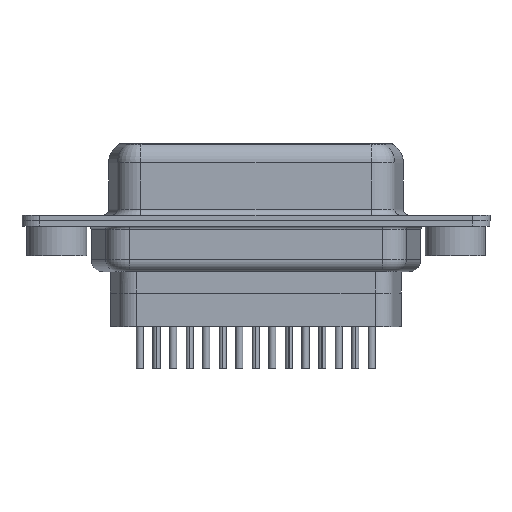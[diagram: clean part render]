
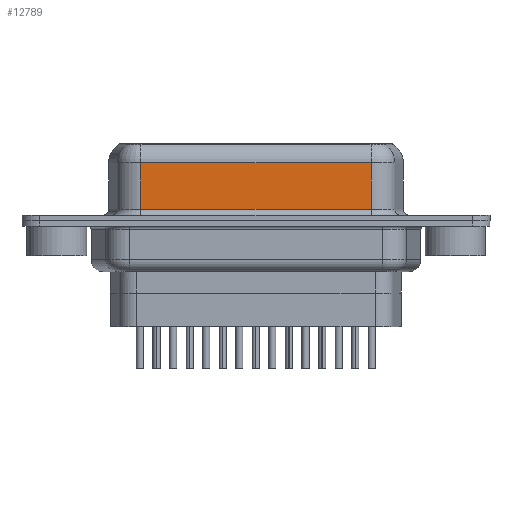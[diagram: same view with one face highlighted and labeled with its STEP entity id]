
A CAD part, front view. The second image highlights one B-rep face of the part: STEP entity #12789.
In plain terms, the highlighted planar face has unit normal (0, -1, 0).
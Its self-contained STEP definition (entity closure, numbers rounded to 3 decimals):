
#417 = ORIENTED_EDGE ( 'NONE', *, *, #6858, .T. ) ;
#1581 = VERTEX_POINT ( 'NONE', #16875 ) ;
#2414 = VERTEX_POINT ( 'NONE', #3272 ) ;
#3272 = CARTESIAN_POINT ( 'NONE',  ( 7.023, -3.95, 0.95 ) ) ;
#3431 = DIRECTION ( 'NONE',  ( -1., 0., 0. ) ) ;
#3705 = CARTESIAN_POINT ( 'NONE',  ( 26.297, -3.95, 4.85 ) ) ;
#6474 = CARTESIAN_POINT ( 'NONE',  ( 26.297, -3.95, 6.6 ) ) ;
#6818 = DIRECTION ( 'NONE',  ( 1., 0., 0. ) ) ;
#6858 = EDGE_CURVE ( 'NONE', #17644, #1581, #11317, .T. ) ;
#7338 = EDGE_CURVE ( 'NONE', #2414, #22537, #8996, .T. ) ;
#7809 = CARTESIAN_POINT ( 'NONE',  ( 7.023, -3.95, 6.6 ) ) ;
#8597 = DIRECTION ( 'NONE',  ( 0., 1., 0. ) ) ;
#8996 = LINE ( 'NONE', #24729, #21390 ) ;
#9971 = EDGE_CURVE ( 'NONE', #1581, #2414, #13467, .T. ) ;
#10147 = ORIENTED_EDGE ( 'NONE', *, *, #7338, .T. ) ;
#10273 = VECTOR ( 'NONE', #3431, 1000. ) ;
#10531 = FACE_OUTER_BOUND ( 'NONE', #23158, .T. ) ;
#11317 = LINE ( 'NONE', #3705, #10273 ) ;
#11361 = CARTESIAN_POINT ( 'NONE',  ( 26.297, -3.95, 4.85 ) ) ;
#11907 = CARTESIAN_POINT ( 'NONE',  ( 26.297, -3.95, 0.95 ) ) ;
#12156 = DIRECTION ( 'NONE',  ( 0., 0., -1. ) ) ;
#12589 = DIRECTION ( 'NONE',  ( 0., 0., 1. ) ) ;
#12789 = ADVANCED_FACE ( 'NONE', ( #10531 ), #24206, .F. ) ;
#13467 = LINE ( 'NONE', #7809, #23481 ) ;
#14210 = LINE ( 'NONE', #6474, #17916 ) ;
#14386 = CARTESIAN_POINT ( 'NONE',  ( 26.297, -3.95, 6.6 ) ) ;
#14993 = AXIS2_PLACEMENT_3D ( 'NONE', #14386, #8597, #12589 ) ;
#16875 = CARTESIAN_POINT ( 'NONE',  ( 7.023, -3.95, 4.85 ) ) ;
#17644 = VERTEX_POINT ( 'NONE', #11361 ) ;
#17916 = VECTOR ( 'NONE', #12156, 1000. ) ;
#20847 = EDGE_CURVE ( 'NONE', #17644, #22537, #14210, .T. ) ;
#21390 = VECTOR ( 'NONE', #6818, 1000. ) ;
#21485 = ORIENTED_EDGE ( 'NONE', *, *, #20847, .F. ) ;
#22537 = VERTEX_POINT ( 'NONE', #11907 ) ;
#23158 = EDGE_LOOP ( 'NONE', ( #21485, #417, #25002, #10147 ) ) ;
#23397 = DIRECTION ( 'NONE',  ( 0., 0., -1. ) ) ;
#23481 = VECTOR ( 'NONE', #23397, 1000. ) ;
#24206 = PLANE ( 'NONE',  #14993 ) ;
#24729 = CARTESIAN_POINT ( 'NONE',  ( 26.297, -3.95, 0.95 ) ) ;
#25002 = ORIENTED_EDGE ( 'NONE', *, *, #9971, .T. ) ;
